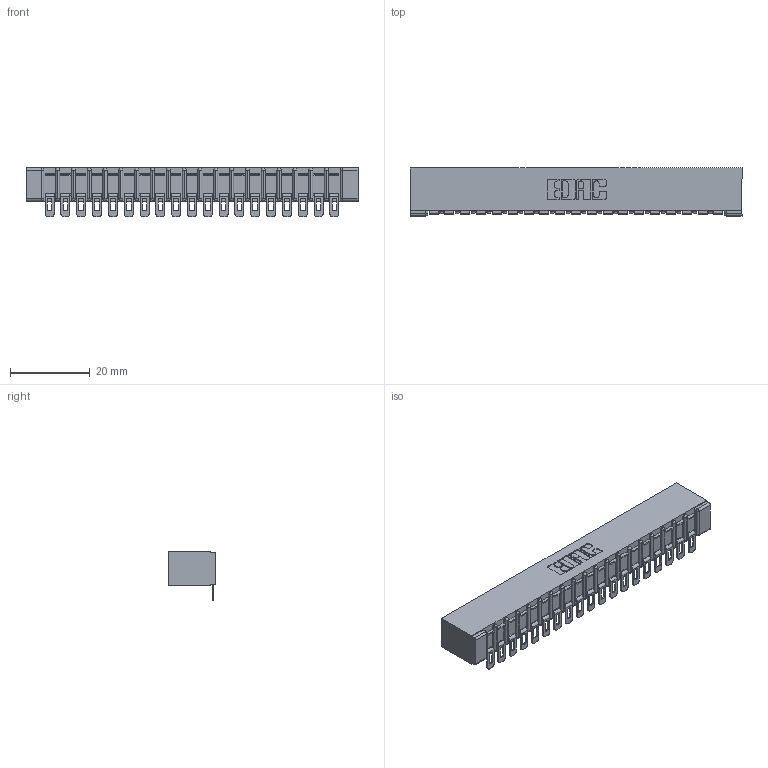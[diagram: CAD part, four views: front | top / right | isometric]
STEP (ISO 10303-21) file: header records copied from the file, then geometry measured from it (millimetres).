
FILE_DESCRIPTION (( 'STEP AP203' ), '1' );
FILE_NAME ('357-019-454-101.STEP', '2020-10-01T02:43:54', ( '' ), ( '' ), 'SwSTEP 2.0', 'SolidWorks 2020', '' );
FILE_SCHEMA (( 'CONFIG_CONTROL_DESIGN' ));
Length unit declared in the file: inch
Products named in the file (3): 357-019-454-101; 307 Part_No Mounting Lugs; 307-290-002_554
Assembly tree (20 placements, depth 2):
  357-019-454-101
    307 Part_No Mounting Lugs
    307-290-002_554  x19
Bounding box: 83.16 x 12.01 x 12.52 mm (x, y, z)
Volume: 5737.6 mm3; surface area: 10854.3 mm2
Topology: 20 solids, 20 shells, 1669 faces, 5106 edges, 3348 vertices
Faces by surface type: plane 940, cylinder 689, sphere 40
Entity records: 19811 total; most frequent: CARTESIAN_POINT 3338, ORIENTED_EDGE 3328, DIRECTION 3258, EDGE_CURVE 1664, LINE 1258, VECTOR 1258, VERTEX_POINT 1080, AXIS2_PLACEMENT_3D 1000
